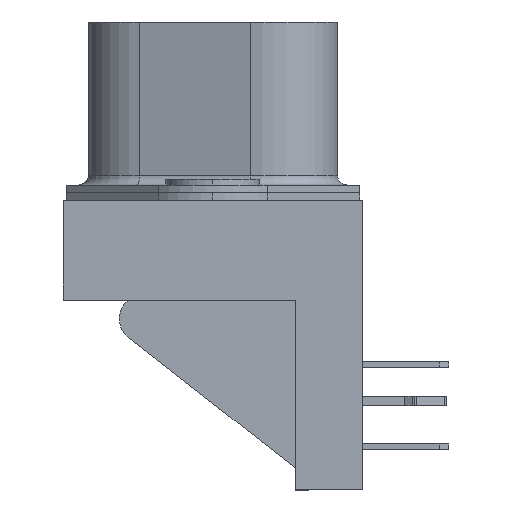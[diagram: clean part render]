
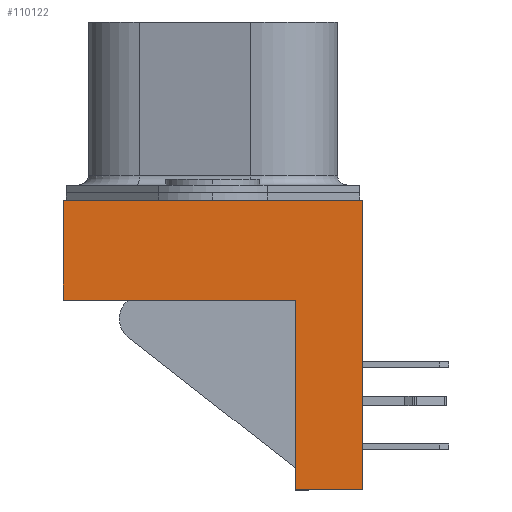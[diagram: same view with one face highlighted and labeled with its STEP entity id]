
A CAD part, left-side view. The second image highlights one B-rep face of the part: STEP entity #110122.
In plain terms, the highlighted planar face has unit normal (-1, 0, 0).
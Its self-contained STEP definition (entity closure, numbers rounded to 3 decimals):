
#1653 = ORIENTED_EDGE ( 'NONE', *, *, #120379, .F. ) ;
#12180 = EDGE_CURVE ( 'NONE', #116365, #43532, #139887, .T. ) ;
#14266 = DIRECTION ( 'NONE',  ( -1., 0., 0. ) ) ;
#16862 = ORIENTED_EDGE ( 'NONE', *, *, #122306, .F. ) ;
#27422 = VERTEX_POINT ( 'NONE', #52699 ) ;
#31937 = LINE ( 'NONE', #114329, #45547 ) ;
#33797 = CARTESIAN_POINT ( 'NONE',  ( -4.125, -4.3, -5.2 ) ) ;
#43532 = VERTEX_POINT ( 'NONE', #78388 ) ;
#45547 = VECTOR ( 'NONE', #169902, 1000. ) ;
#46055 = VECTOR ( 'NONE', #108898, 1000. ) ;
#50672 = LINE ( 'NONE', #159977, #121597 ) ;
#52699 = CARTESIAN_POINT ( 'NONE',  ( -4.125, -4.3, -15.1 ) ) ;
#58412 = CARTESIAN_POINT ( 'NONE',  ( -4.125, 7.8, 0. ) ) ;
#59542 = AXIS2_PLACEMENT_3D ( 'NONE', #111875, #14266, #81528 ) ;
#62668 = VECTOR ( 'NONE', #106572, 1000. ) ;
#63358 = CARTESIAN_POINT ( 'NONE',  ( -4.125, 7.8, -5.2 ) ) ;
#63829 = EDGE_CURVE ( 'NONE', #89635, #43532, #160938, .T. ) ;
#64519 = ORIENTED_EDGE ( 'NONE', *, *, #12180, .F. ) ;
#65002 = DIRECTION ( 'NONE',  ( 0., -1., 0. ) ) ;
#67216 = PLANE ( 'NONE',  #59542 ) ;
#68497 = ORIENTED_EDGE ( 'NONE', *, *, #136423, .T. ) ;
#70291 = ORIENTED_EDGE ( 'NONE', *, *, #63829, .T. ) ;
#77053 = LINE ( 'NONE', #160367, #62668 ) ;
#78388 = CARTESIAN_POINT ( 'NONE',  ( -4.125, -7.8, 0. ) ) ;
#79536 = VERTEX_POINT ( 'NONE', #33797 ) ;
#81528 = DIRECTION ( 'NONE',  ( 0., -1., 0. ) ) ;
#84632 = EDGE_LOOP ( 'NONE', ( #164065, #16862, #68497, #70291, #64519, #1653 ) ) ;
#89635 = VERTEX_POINT ( 'NONE', #154612 ) ;
#92826 = VECTOR ( 'NONE', #93359, 1000. ) ;
#93359 = DIRECTION ( 'NONE',  ( 0., 1., 0. ) ) ;
#94952 = FACE_OUTER_BOUND ( 'NONE', #84632, .T. ) ;
#96478 = VERTEX_POINT ( 'NONE', #63358 ) ;
#104320 = EDGE_CURVE ( 'NONE', #79536, #96478, #148882, .T. ) ;
#106572 = DIRECTION ( 'NONE',  ( 0., 0., 1. ) ) ;
#108898 = DIRECTION ( 'NONE',  ( 0., 0., 1. ) ) ;
#110122 = ADVANCED_FACE ( 'NONE', ( #94952 ), #67216, .T. ) ;
#111875 = CARTESIAN_POINT ( 'NONE',  ( -4.125, 7.8, -15.1 ) ) ;
#114329 = CARTESIAN_POINT ( 'NONE',  ( -4.125, -4.3, -15.1 ) ) ;
#116365 = VERTEX_POINT ( 'NONE', #134510 ) ;
#120379 = EDGE_CURVE ( 'NONE', #96478, #116365, #77053, .T. ) ;
#121597 = VECTOR ( 'NONE', #65002, 1000. ) ;
#122306 = EDGE_CURVE ( 'NONE', #27422, #79536, #31937, .T. ) ;
#134510 = CARTESIAN_POINT ( 'NONE',  ( -4.125, 7.8, 0. ) ) ;
#136423 = EDGE_CURVE ( 'NONE', #27422, #89635, #50672, .T. ) ;
#139887 = LINE ( 'NONE', #58412, #140625 ) ;
#140625 = VECTOR ( 'NONE', #163292, 1000. ) ;
#148882 = LINE ( 'NONE', #176671, #92826 ) ;
#154612 = CARTESIAN_POINT ( 'NONE',  ( -4.125, -7.8, -15.1 ) ) ;
#159977 = CARTESIAN_POINT ( 'NONE',  ( -4.125, 7.8, -15.1 ) ) ;
#160367 = CARTESIAN_POINT ( 'NONE',  ( -4.125, 7.8, -15.1 ) ) ;
#160938 = LINE ( 'NONE', #162702, #46055 ) ;
#162702 = CARTESIAN_POINT ( 'NONE',  ( -4.125, -7.8, -15.1 ) ) ;
#163292 = DIRECTION ( 'NONE',  ( 0., -1., 0. ) ) ;
#164065 = ORIENTED_EDGE ( 'NONE', *, *, #104320, .F. ) ;
#169902 = DIRECTION ( 'NONE',  ( 0., 0., 1. ) ) ;
#176671 = CARTESIAN_POINT ( 'NONE',  ( -4.125, 7.8, -5.2 ) ) ;
